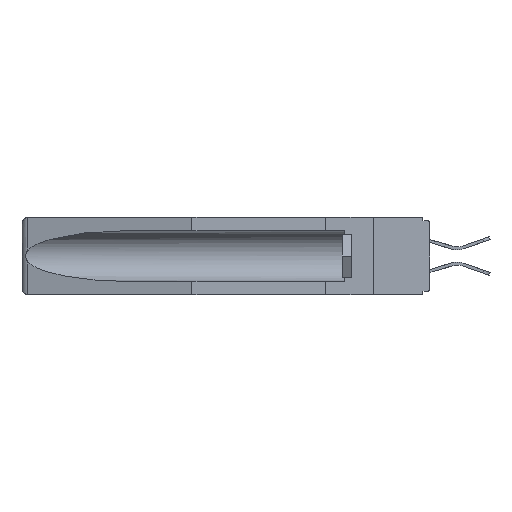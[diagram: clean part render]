
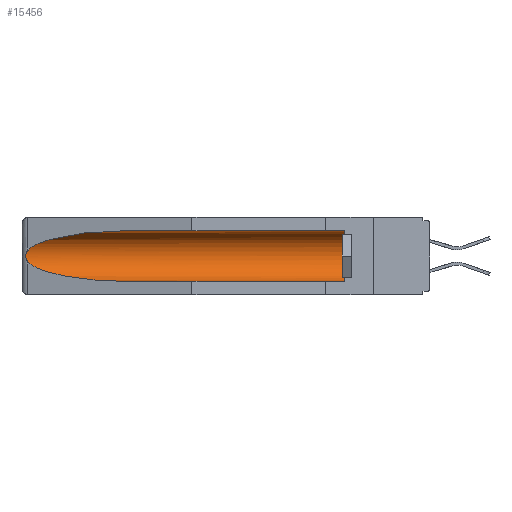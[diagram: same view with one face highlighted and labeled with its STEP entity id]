
A CAD part, left-side view. The second image highlights one B-rep face of the part: STEP entity #15456.
In plain terms, the highlighted cylindrical face has radius 2.857 mm (diameter 5.715 mm), a partial arc.
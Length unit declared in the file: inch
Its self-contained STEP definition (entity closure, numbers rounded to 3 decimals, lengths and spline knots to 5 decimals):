
#77 = FACE_OUTER_BOUND ( 'NONE', #9936, .T. ) ;
#326 = CARTESIAN_POINT ( 'NONE',  ( 0.25451, 1.48313, -0.24835 ) ) ;
#652 = CARTESIAN_POINT ( 'NONE',  ( 0.155, 1.07973, -0.059 ) ) ;
#775 = CARTESIAN_POINT ( 'NONE',  ( 0.155, 0.126, -0.1715 ) ) ;
#1095 = DIRECTION ( 'NONE',  ( 0., 1., 0. ) ) ;
#1163 = ORIENTED_EDGE ( 'NONE', *, *, #8944, .T. ) ;
#1901 = EDGE_CURVE ( 'NONE', #14976, #2370, #10280, .T. ) ;
#2148 = VECTOR ( 'NONE', #6791, 39.37008 ) ;
#2248 = CARTESIAN_POINT ( 'NONE',  ( 0.21114, 1.30732, -0.059 ) ) ;
#2370 = VERTEX_POINT ( 'NONE', #15533 ) ;
#2591 = ORIENTED_EDGE ( 'NONE', *, *, #18160, .T. ) ;
#2615 = AXIS2_PLACEMENT_3D ( 'NONE', #16839, #16650, #7681 ) ;
#3181 = ORIENTED_EDGE ( 'NONE', *, *, #1901, .F. ) ;
#3521 = CARTESIAN_POINT ( 'NONE',  ( 0.26537, 1.52718, -0.14972 ) ) ;
#3768 = VERTEX_POINT ( 'NONE', #12898 ) ;
#4083 = AXIS2_PLACEMENT_3D ( 'NONE', #775, #11302, #8354 ) ;
#4782 = CARTESIAN_POINT ( 'NONE',  ( 0.26537, 1.52718, -0.19328 ) ) ;
#5101 = CARTESIAN_POINT ( 'NONE',  ( 0.155, 1.07973, -0.059 ) ) ;
#5210 = CARTESIAN_POINT ( 'NONE',  ( 0.155, -0.30754, -0.284 ) ) ;
#5238 = CARTESIAN_POINT ( 'NONE',  ( 0.25451, 1.48313, -0.09465 ) ) ;
#5870 = EDGE_CURVE ( 'NONE', #17248, #2370, #12185, .T. ) ;
#6436 = CARTESIAN_POINT ( 'NONE',  ( 0.155, 0.126, -0.284 ) ) ;
#6791 = DIRECTION ( 'NONE',  ( 0., 1., 0. ) ) ;
#7010 = CARTESIAN_POINT ( 'NONE',  ( 0.26537, 1.52718, -0.14972 ) ) ;
#7158 =( BOUNDED_CURVE ( )  B_SPLINE_CURVE ( 3, ( #652, #2248, #5238, #3521 ),
 .UNSPECIFIED., .F., .F. ) 
 B_SPLINE_CURVE_WITH_KNOTS ( ( 4, 4 ),
 ( 4.71239, 6.08839 ),
 .UNSPECIFIED. ) 
 CURVE ( )  GEOMETRIC_REPRESENTATION_ITEM ( )  RATIONAL_B_SPLINE_CURVE ( ( 1., 0.848, 0.848, 1. ) ) 
 REPRESENTATION_ITEM ( '' )  );
#7276 = VECTOR ( 'NONE', #1095, 39.37008 ) ;
#7342 = ORIENTED_EDGE ( 'NONE', *, *, #5870, .T. ) ;
#7462 = CYLINDRICAL_SURFACE ( 'NONE', #2615, 0.1125 ) ;
#7681 = DIRECTION ( 'NONE',  ( 0., 0., 1. ) ) ;
#7762 = EDGE_CURVE ( 'NONE', #3768, #17248, #8892, .T. ) ;
#8297 = ORIENTED_EDGE ( 'NONE', *, *, #7762, .T. ) ;
#8354 = DIRECTION ( 'NONE',  ( 0., 0., 1. ) ) ;
#8561 = CARTESIAN_POINT ( 'NONE',  ( 0.2675, 1.53308, -0.16763 ) ) ;
#8892 = B_SPLINE_CURVE_WITH_KNOTS ( 'NONE', 3,
 ( #7010, #13331, #17826, #17687, #8561, #19462, #11702, #19201, #11629, #16453 ),
 .UNSPECIFIED., .F., .F.,
 ( 4, 2, 2, 2, 4 ),
 ( 0., 0.00029, 0.00058, 0.00087, 0.00117 ),
 .UNSPECIFIED. ) ;
#8944 = EDGE_CURVE ( 'NONE', #18295, #11333, #15904, .T. ) ;
#9936 = EDGE_LOOP ( 'NONE', ( #2591, #8297, #7342, #3181, #10526, #1163 ) ) ;
#10280 = LINE ( 'NONE', #5210, #2148 ) ;
#10446 = CARTESIAN_POINT ( 'NONE',  ( 0.155, -0.30754, -0.059 ) ) ;
#10526 = ORIENTED_EDGE ( 'NONE', *, *, #18933, .T. ) ;
#10874 = CARTESIAN_POINT ( 'NONE',  ( 0.155, 1.07973, -0.284 ) ) ;
#11302 = DIRECTION ( 'NONE',  ( 0., -1., 0. ) ) ;
#11333 = VERTEX_POINT ( 'NONE', #5101 ) ;
#11629 = CARTESIAN_POINT ( 'NONE',  ( 0.26597, 1.5296, -0.19026 ) ) ;
#11702 = CARTESIAN_POINT ( 'NONE',  ( 0.2673, 1.53269, -0.17917 ) ) ;
#12185 =( BOUNDED_CURVE ( )  B_SPLINE_CURVE ( 3, ( #4782, #326, #12268, #10874 ),
 .UNSPECIFIED., .F., .F. ) 
 B_SPLINE_CURVE_WITH_KNOTS ( ( 4, 4 ),
 ( 0.1948, 1.5708 ),
 .UNSPECIFIED. ) 
 CURVE ( )  GEOMETRIC_REPRESENTATION_ITEM ( )  RATIONAL_B_SPLINE_CURVE ( ( 1., 0.848, 0.848, 1. ) ) 
 REPRESENTATION_ITEM ( '' )  );
#12268 = CARTESIAN_POINT ( 'NONE',  ( 0.21114, 1.30732, -0.284 ) ) ;
#12898 = CARTESIAN_POINT ( 'NONE',  ( 0.26537, 1.52718, -0.14972 ) ) ;
#13025 = CARTESIAN_POINT ( 'NONE',  ( 0.155, 0.126, -0.059 ) ) ;
#13331 = CARTESIAN_POINT ( 'NONE',  ( 0.26597, 1.52961, -0.15275 ) ) ;
#14976 = VERTEX_POINT ( 'NONE', #6436 ) ;
#15456 = ADVANCED_FACE ( 'NONE', ( #77 ), #7462, .F. ) ;
#15533 = CARTESIAN_POINT ( 'NONE',  ( 0.155, 1.07973, -0.284 ) ) ;
#15904 = LINE ( 'NONE', #10446, #7276 ) ;
#15976 = CIRCLE ( 'NONE', #4083, 0.1125 ) ;
#16453 = CARTESIAN_POINT ( 'NONE',  ( 0.26537, 1.52718, -0.19328 ) ) ;
#16650 = DIRECTION ( 'NONE',  ( 0., 1., 0. ) ) ;
#16839 = CARTESIAN_POINT ( 'NONE',  ( 0.155, -0.30754, -0.1715 ) ) ;
#17248 = VERTEX_POINT ( 'NONE', #19643 ) ;
#17687 = CARTESIAN_POINT ( 'NONE',  ( 0.2673, 1.5327, -0.16383 ) ) ;
#17826 = CARTESIAN_POINT ( 'NONE',  ( 0.26654, 1.53092, -0.15636 ) ) ;
#18160 = EDGE_CURVE ( 'NONE', #11333, #3768, #7158, .T. ) ;
#18295 = VERTEX_POINT ( 'NONE', #13025 ) ;
#18933 = EDGE_CURVE ( 'NONE', #14976, #18295, #15976, .T. ) ;
#19201 = CARTESIAN_POINT ( 'NONE',  ( 0.26655, 1.53094, -0.18657 ) ) ;
#19462 = CARTESIAN_POINT ( 'NONE',  ( 0.2675, 1.53308, -0.17534 ) ) ;
#19643 = CARTESIAN_POINT ( 'NONE',  ( 0.26537, 1.52718, -0.19328 ) ) ;
